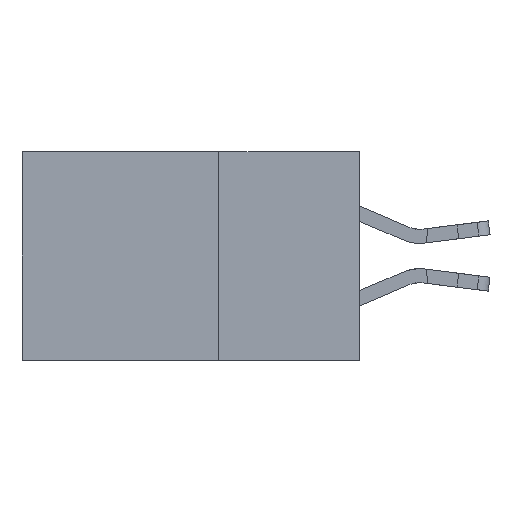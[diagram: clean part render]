
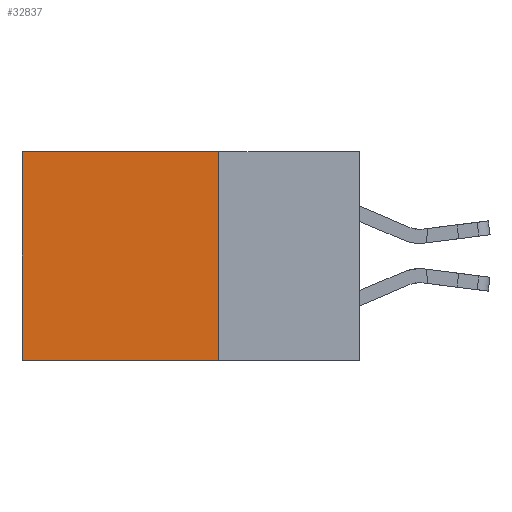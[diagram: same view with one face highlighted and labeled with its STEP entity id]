
A CAD part, left-side view. The second image highlights one B-rep face of the part: STEP entity #32837.
In plain terms, the highlighted planar face has unit normal (-1, 0, 0).
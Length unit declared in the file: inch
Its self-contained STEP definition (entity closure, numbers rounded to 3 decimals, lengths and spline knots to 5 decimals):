
#1547 = VERTEX_POINT ( 'NONE', #21294 ) ;
#2005 = ORIENTED_EDGE ( 'NONE', *, *, #6262, .F. ) ;
#2172 = ORIENTED_EDGE ( 'NONE', *, *, #8603, .T. ) ;
#2213 = VECTOR ( 'NONE', #14743, 39.37008 ) ;
#2431 = ORIENTED_EDGE ( 'NONE', *, *, #12186, .F. ) ;
#3920 = PLANE ( 'NONE',  #10820 ) ;
#4047 = VECTOR ( 'NONE', #15640, 39.37008 ) ;
#6262 = EDGE_CURVE ( 'NONE', #21323, #24298, #10145, .T. ) ;
#6716 = VERTEX_POINT ( 'NONE', #15767 ) ;
#7344 = ORIENTED_EDGE ( 'NONE', *, *, #31261, .T. ) ;
#8084 = CARTESIAN_POINT ( 'NONE',  ( 0.2875, 0.6, 0. ) ) ;
#8603 = EDGE_CURVE ( 'NONE', #6716, #1547, #30050, .T. ) ;
#9296 = CARTESIAN_POINT ( 'NONE',  ( 0.2875, 0.25, 0. ) ) ;
#10145 = LINE ( 'NONE', #31736, #4047 ) ;
#10820 = AXIS2_PLACEMENT_3D ( 'NONE', #13774, #32365, #24578 ) ;
#12186 = EDGE_CURVE ( 'NONE', #24298, #1547, #28380, .T. ) ;
#13597 = FACE_OUTER_BOUND ( 'NONE', #25239, .T. ) ;
#13774 = CARTESIAN_POINT ( 'NONE',  ( 0.2875, 0.25, 0. ) ) ;
#14743 = DIRECTION ( 'NONE',  ( 0., 1., 0. ) ) ;
#15640 = DIRECTION ( 'NONE',  ( 0., 0., -1. ) ) ;
#15767 = CARTESIAN_POINT ( 'NONE',  ( 0.2875, 0.6, 0. ) ) ;
#16152 = CARTESIAN_POINT ( 'NONE',  ( 0.2875, 0.25, 0. ) ) ;
#19749 = VECTOR ( 'NONE', #23106, 39.37008 ) ;
#21294 = CARTESIAN_POINT ( 'NONE',  ( 0.2875, 0.6, -0.37 ) ) ;
#21323 = VERTEX_POINT ( 'NONE', #16152 ) ;
#22396 = VECTOR ( 'NONE', #27563, 39.37008 ) ;
#23106 = DIRECTION ( 'NONE',  ( 0., 1., 0. ) ) ;
#24298 = VERTEX_POINT ( 'NONE', #31435 ) ;
#24578 = DIRECTION ( 'NONE',  ( 0., 0., -1. ) ) ;
#25239 = EDGE_LOOP ( 'NONE', ( #2172, #2431, #2005, #7344 ) ) ;
#27563 = DIRECTION ( 'NONE',  ( 0., 0., -1. ) ) ;
#28380 = LINE ( 'NONE', #31208, #2213 ) ;
#30050 = LINE ( 'NONE', #8084, #22396 ) ;
#31079 = LINE ( 'NONE', #9296, #19749 ) ;
#31208 = CARTESIAN_POINT ( 'NONE',  ( 0.2875, 0.25, -0.37 ) ) ;
#31261 = EDGE_CURVE ( 'NONE', #21323, #6716, #31079, .T. ) ;
#31435 = CARTESIAN_POINT ( 'NONE',  ( 0.2875, 0.25, -0.37 ) ) ;
#31736 = CARTESIAN_POINT ( 'NONE',  ( 0.2875, 0.25, 0. ) ) ;
#32365 = DIRECTION ( 'NONE',  ( 1., 0., 0. ) ) ;
#32837 = ADVANCED_FACE ( 'NONE', ( #13597 ), #3920, .F. ) ;
